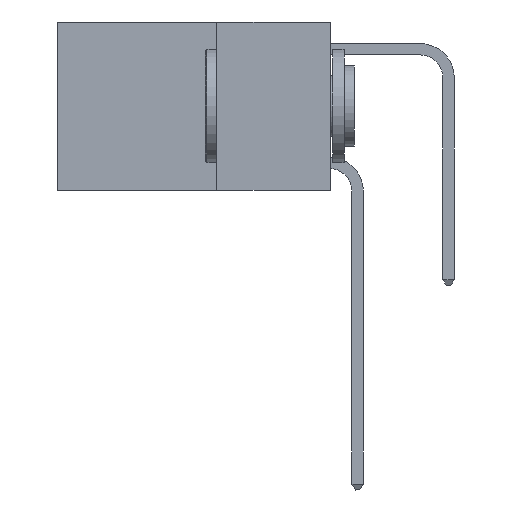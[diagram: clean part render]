
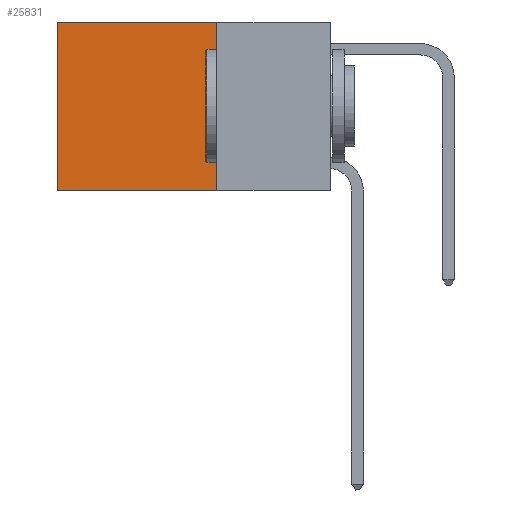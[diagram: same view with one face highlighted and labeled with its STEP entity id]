
A CAD part, left-side view. The second image highlights one B-rep face of the part: STEP entity #25831.
In plain terms, the highlighted planar face has unit normal (-1, 0, 0).
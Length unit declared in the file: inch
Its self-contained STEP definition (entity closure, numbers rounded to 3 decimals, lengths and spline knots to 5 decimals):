
#362 = VECTOR ( 'NONE', #2499, 39.37008 ) ;
#682 = AXIS2_PLACEMENT_3D ( 'NONE', #8341, #15440, #25756 ) ;
#2256 = VERTEX_POINT ( 'NONE', #3552 ) ;
#2499 = DIRECTION ( 'NONE',  ( 0., 1., 0. ) ) ;
#3552 = CARTESIAN_POINT ( 'NONE',  ( 0.2625, 0.6, 0. ) ) ;
#4563 = DIRECTION ( 'NONE',  ( 0., 0., -1. ) ) ;
#5064 = CARTESIAN_POINT ( 'NONE',  ( 0.2625, 0.25, -0.37 ) ) ;
#5219 = CARTESIAN_POINT ( 'NONE',  ( 0.2625, 0.25, 0. ) ) ;
#6378 = VECTOR ( 'NONE', #32449, 39.37008 ) ;
#7781 = VERTEX_POINT ( 'NONE', #25986 ) ;
#8014 = FACE_OUTER_BOUND ( 'NONE', #10709, .T. ) ;
#8341 = CARTESIAN_POINT ( 'NONE',  ( 0.2625, 0.25, 0. ) ) ;
#10339 = LINE ( 'NONE', #17410, #19096 ) ;
#10709 = EDGE_LOOP ( 'NONE', ( #14480, #24795, #19075, #19714 ) ) ;
#11688 = CARTESIAN_POINT ( 'NONE',  ( 0.2625, 0.25, 0. ) ) ;
#11856 = LINE ( 'NONE', #22133, #6378 ) ;
#13082 = PLANE ( 'NONE',  #682 ) ;
#14480 = ORIENTED_EDGE ( 'NONE', *, *, #23932, .T. ) ;
#15440 = DIRECTION ( 'NONE',  ( 1., 0., 0. ) ) ;
#17410 = CARTESIAN_POINT ( 'NONE',  ( 0.2625, 0.25, 0. ) ) ;
#17454 = VERTEX_POINT ( 'NONE', #5064 ) ;
#17680 = DIRECTION ( 'NONE',  ( 0., 0., -1. ) ) ;
#17921 = VECTOR ( 'NONE', #17680, 39.37008 ) ;
#19075 = ORIENTED_EDGE ( 'NONE', *, *, #28544, .F. ) ;
#19096 = VECTOR ( 'NONE', #4563, 39.37008 ) ;
#19547 = EDGE_CURVE ( 'NONE', #17454, #7781, #11856, .T. ) ;
#19714 = ORIENTED_EDGE ( 'NONE', *, *, #32397, .T. ) ;
#20205 = LINE ( 'NONE', #32886, #17921 ) ;
#22133 = CARTESIAN_POINT ( 'NONE',  ( 0.2625, 0.25, -0.37 ) ) ;
#23932 = EDGE_CURVE ( 'NONE', #2256, #7781, #20205, .T. ) ;
#24795 = ORIENTED_EDGE ( 'NONE', *, *, #19547, .F. ) ;
#25678 = LINE ( 'NONE', #5219, #362 ) ;
#25756 = DIRECTION ( 'NONE',  ( 0., 0., -1. ) ) ;
#25831 = ADVANCED_FACE ( 'NONE', ( #8014 ), #13082, .F. ) ;
#25986 = CARTESIAN_POINT ( 'NONE',  ( 0.2625, 0.6, -0.37 ) ) ;
#28544 = EDGE_CURVE ( 'NONE', #32160, #17454, #10339, .T. ) ;
#32160 = VERTEX_POINT ( 'NONE', #11688 ) ;
#32397 = EDGE_CURVE ( 'NONE', #32160, #2256, #25678, .T. ) ;
#32449 = DIRECTION ( 'NONE',  ( 0., 1., 0. ) ) ;
#32886 = CARTESIAN_POINT ( 'NONE',  ( 0.2625, 0.6, 0. ) ) ;
